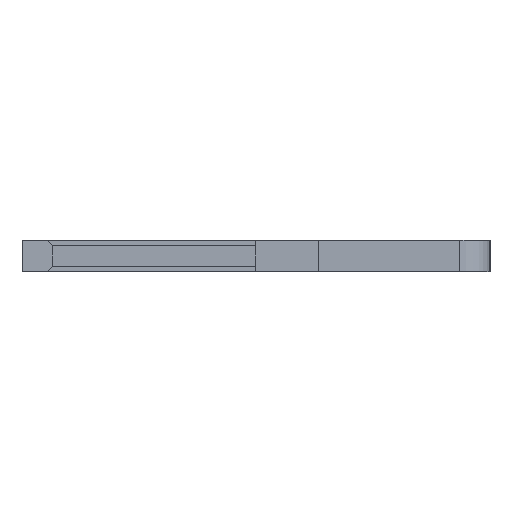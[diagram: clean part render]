
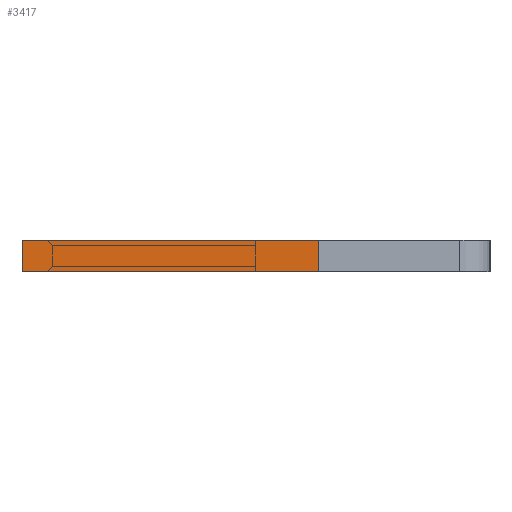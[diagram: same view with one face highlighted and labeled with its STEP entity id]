
A CAD part, left-side view. The second image highlights one B-rep face of the part: STEP entity #3417.
In plain terms, the highlighted face is planar.
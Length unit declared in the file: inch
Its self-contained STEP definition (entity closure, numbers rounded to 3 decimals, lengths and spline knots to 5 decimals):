
#19 = CARTESIAN_POINT ( 'NONE',  ( -0.01, 0.15, -0.04 ) ) ;
#196 = CARTESIAN_POINT ( 'NONE',  ( 0.01, 0.15, -0.04 ) ) ;
#202 = EDGE_CURVE ( 'NONE', #3512, #1582, #3495, .T. ) ;
#265 = DIRECTION ( 'NONE',  ( -1., 0., 0. ) ) ;
#644 = VECTOR ( 'NONE', #2911, 39.37008 ) ;
#685 = DIRECTION ( 'NONE',  ( 0., 1., 0. ) ) ;
#871 = DIRECTION ( 'NONE',  ( 0., 1., 0. ) ) ;
#939 = EDGE_CURVE ( 'NONE', #3512, #2362, #3331, .T. ) ;
#1434 = ORIENTED_EDGE ( 'NONE', *, *, #4294, .T. ) ;
#1462 = ORIENTED_EDGE ( 'NONE', *, *, #202, .T. ) ;
#1582 = VERTEX_POINT ( 'NONE', #1862 ) ;
#1586 = DIRECTION ( 'NONE',  ( 1., 0., 0. ) ) ;
#1653 = LINE ( 'NONE', #4184, #2710 ) ;
#1775 = CARTESIAN_POINT ( 'NONE',  ( 0.01, -0.04, -0.04 ) ) ;
#1862 = CARTESIAN_POINT ( 'NONE',  ( -0.01, -0.04, -0.04 ) ) ;
#2014 = PLANE ( 'NONE',  #3723 ) ;
#2254 = ORIENTED_EDGE ( 'NONE', *, *, #939, .F. ) ;
#2259 = FACE_OUTER_BOUND ( 'NONE', #3748, .T. ) ;
#2362 = VERTEX_POINT ( 'NONE', #196 ) ;
#2710 = VECTOR ( 'NONE', #265, 39.37008 ) ;
#2830 = EDGE_CURVE ( 'NONE', #2362, #3490, #1653, .T. ) ;
#2911 = DIRECTION ( 'NONE',  ( -1., 0., 0. ) ) ;
#3081 = CARTESIAN_POINT ( 'NONE',  ( -0.01, 0.15, -0.04 ) ) ;
#3142 = CARTESIAN_POINT ( 'NONE',  ( 0.01, 0.15, -0.04 ) ) ;
#3253 = VECTOR ( 'NONE', #685, 39.37008 ) ;
#3323 = CARTESIAN_POINT ( 'NONE',  ( 0.01, 0.15, -0.04 ) ) ;
#3331 = LINE ( 'NONE', #3323, #4021 ) ;
#3417 = ADVANCED_FACE ( 'NONE', ( #2259 ), #2014, .F. ) ;
#3490 = VERTEX_POINT ( 'NONE', #3081 ) ;
#3495 = LINE ( 'NONE', #1775, #644 ) ;
#3512 = VERTEX_POINT ( 'NONE', #3914 ) ;
#3723 = AXIS2_PLACEMENT_3D ( 'NONE', #3142, #4231, #1586 ) ;
#3748 = EDGE_LOOP ( 'NONE', ( #1434, #3994, #2254, #1462 ) ) ;
#3869 = LINE ( 'NONE', #19, #3253 ) ;
#3914 = CARTESIAN_POINT ( 'NONE',  ( 0.01, -0.04, -0.04 ) ) ;
#3994 = ORIENTED_EDGE ( 'NONE', *, *, #2830, .F. ) ;
#4021 = VECTOR ( 'NONE', #871, 39.37008 ) ;
#4184 = CARTESIAN_POINT ( 'NONE',  ( 0.01, 0.15, -0.04 ) ) ;
#4231 = DIRECTION ( 'NONE',  ( 0., 0., 1. ) ) ;
#4294 = EDGE_CURVE ( 'NONE', #1582, #3490, #3869, .T. ) ;
